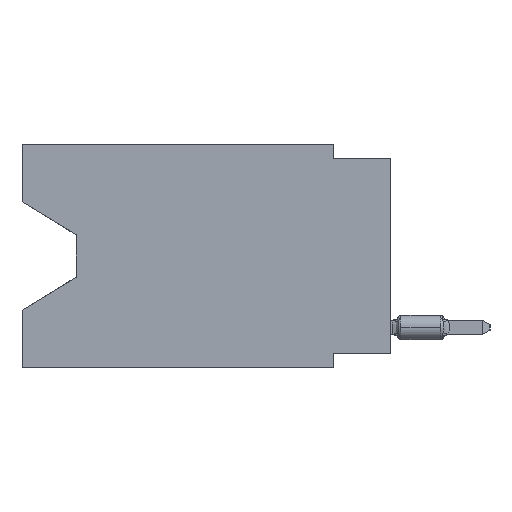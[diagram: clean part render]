
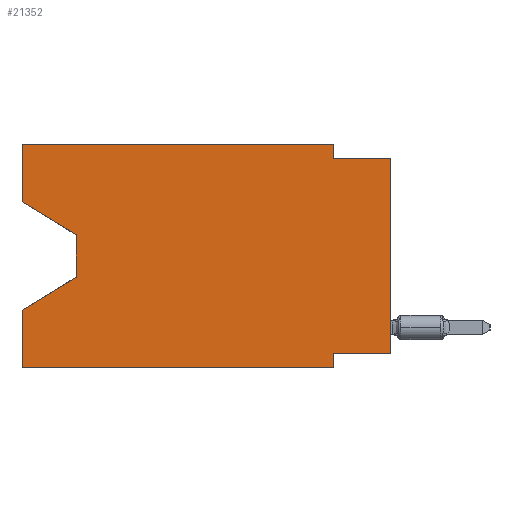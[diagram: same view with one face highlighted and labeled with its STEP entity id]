
A CAD part, left-side view. The second image highlights one B-rep face of the part: STEP entity #21352.
In plain terms, the highlighted planar face has unit normal (-1, 0, 0).
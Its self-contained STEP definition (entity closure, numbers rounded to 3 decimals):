
#1010 = VECTOR ( 'NONE', #30172, 1000. ) ;
#1150 = ORIENTED_EDGE ( 'NONE', *, *, #23051, .T. ) ;
#1176 = DIRECTION ( 'NONE',  ( 0., 0., 1. ) ) ;
#1302 = DIRECTION ( 'NONE',  ( 0., 0., 1. ) ) ;
#1735 = CARTESIAN_POINT ( 'NONE',  ( 0., 0., 0. ) ) ;
#2329 = EDGE_CURVE ( 'NONE', #19913, #29093, #39961, .T. ) ;
#2460 = CARTESIAN_POINT ( 'NONE',  ( 0., 16.383, -2.546 ) ) ;
#2605 = VERTEX_POINT ( 'NONE', #6800 ) ;
#3284 = VECTOR ( 'NONE', #35981, 1000. ) ;
#3631 = LINE ( 'NONE', #40760, #1010 ) ;
#3651 = CARTESIAN_POINT ( 'NONE',  ( 0., 2.54, 0. ) ) ;
#4094 = DIRECTION ( 'NONE',  ( 0., 1., 0. ) ) ;
#4139 = CARTESIAN_POINT ( 'NONE',  ( 0., 2.54, -9.906 ) ) ;
#4316 = VERTEX_POINT ( 'NONE', #26031 ) ;
#4637 = ORIENTED_EDGE ( 'NONE', *, *, #6625, .T. ) ;
#5094 = VECTOR ( 'NONE', #1302, 1000. ) ;
#5247 = EDGE_CURVE ( 'NONE', #20500, #32121, #35694, .T. ) ;
#6625 = EDGE_CURVE ( 'NONE', #19913, #32121, #41486, .T. ) ;
#6800 = CARTESIAN_POINT ( 'NONE',  ( 0., 16.383, -9.906 ) ) ;
#7264 = DIRECTION ( 'NONE',  ( 0., 0., -1. ) ) ;
#7619 = ORIENTED_EDGE ( 'NONE', *, *, #9772, .F. ) ;
#7693 = DIRECTION ( 'NONE',  ( 1., 0., 0. ) ) ;
#7771 = CARTESIAN_POINT ( 'NONE',  ( 0., 16.383, 0. ) ) ;
#7811 = LINE ( 'NONE', #4139, #41850 ) ;
#8236 = DIRECTION ( 'NONE',  ( 0., 0., 1. ) ) ;
#8363 = CARTESIAN_POINT ( 'NONE',  ( 0., 13.97, -5.893 ) ) ;
#8484 = EDGE_CURVE ( 'NONE', #26844, #34857, #31747, .T. ) ;
#8653 = CARTESIAN_POINT ( 'NONE',  ( 0., 16.383, 0. ) ) ;
#8928 = DIRECTION ( 'NONE',  ( 0., -1., 0. ) ) ;
#9772 = EDGE_CURVE ( 'NONE', #34857, #26220, #42355, .T. ) ;
#10543 = CARTESIAN_POINT ( 'NONE',  ( 0., 0., -0.635 ) ) ;
#11163 = LINE ( 'NONE', #14217, #24694 ) ;
#11628 = DIRECTION ( 'NONE',  ( 0., -0.855, -0.519 ) ) ;
#12392 = EDGE_CURVE ( 'NONE', #29044, #34066, #26334, .T. ) ;
#13186 = ORIENTED_EDGE ( 'NONE', *, *, #23347, .F. ) ;
#14217 = CARTESIAN_POINT ( 'NONE',  ( 0., 16.383, 0. ) ) ;
#14349 = EDGE_CURVE ( 'NONE', #2605, #34066, #11163, .T. ) ;
#15320 = CARTESIAN_POINT ( 'NONE',  ( 0., 2.54, -9.271 ) ) ;
#15843 = ORIENTED_EDGE ( 'NONE', *, *, #8484, .F. ) ;
#16494 = CARTESIAN_POINT ( 'NONE',  ( 0., 0., -9.271 ) ) ;
#17186 = ORIENTED_EDGE ( 'NONE', *, *, #35524, .T. ) ;
#17229 = ORIENTED_EDGE ( 'NONE', *, *, #12392, .T. ) ;
#17276 = FACE_OUTER_BOUND ( 'NONE', #36781, .T. ) ;
#17323 = VERTEX_POINT ( 'NONE', #34441 ) ;
#17388 = DIRECTION ( 'NONE',  ( 0., 0., -1. ) ) ;
#18300 = LINE ( 'NONE', #21785, #27297 ) ;
#18641 = EDGE_CURVE ( 'NONE', #26220, #20500, #3631, .T. ) ;
#19153 = ORIENTED_EDGE ( 'NONE', *, *, #14349, .F. ) ;
#19913 = VERTEX_POINT ( 'NONE', #31413 ) ;
#20136 = VECTOR ( 'NONE', #4094, 1000. ) ;
#20457 = ORIENTED_EDGE ( 'NONE', *, *, #18641, .F. ) ;
#20500 = VERTEX_POINT ( 'NONE', #32221 ) ;
#20895 = AXIS2_PLACEMENT_3D ( 'NONE', #30787, #7693, #7264 ) ;
#21352 = ADVANCED_FACE ( 'NONE', ( #17276 ), #37702, .F. ) ;
#21785 = CARTESIAN_POINT ( 'NONE',  ( 0., 16.383, -9.906 ) ) ;
#22021 = VECTOR ( 'NONE', #11628, 1000. ) ;
#22200 = CARTESIAN_POINT ( 'NONE',  ( 0., 16.383, 0. ) ) ;
#22385 = VECTOR ( 'NONE', #29401, 1000. ) ;
#22642 = DIRECTION ( 'NONE',  ( 0., 0.855, -0.519 ) ) ;
#22731 = LINE ( 'NONE', #36618, #3284 ) ;
#22875 = CARTESIAN_POINT ( 'NONE',  ( 0., 0., -0.635 ) ) ;
#23051 = EDGE_CURVE ( 'NONE', #2605, #17323, #18300, .T. ) ;
#23347 = EDGE_CURVE ( 'NONE', #29093, #17323, #7811, .T. ) ;
#24694 = VECTOR ( 'NONE', #1176, 1000. ) ;
#26031 = CARTESIAN_POINT ( 'NONE',  ( 0., 13.97, -4.013 ) ) ;
#26220 = VERTEX_POINT ( 'NONE', #3651 ) ;
#26334 = LINE ( 'NONE', #29168, #30709 ) ;
#26844 = VERTEX_POINT ( 'NONE', #2460 ) ;
#27297 = VECTOR ( 'NONE', #8928, 1000. ) ;
#29037 = LINE ( 'NONE', #34909, #22021 ) ;
#29044 = VERTEX_POINT ( 'NONE', #8363 ) ;
#29093 = VERTEX_POINT ( 'NONE', #15320 ) ;
#29168 = CARTESIAN_POINT ( 'NONE',  ( 0., 13.97, -5.893 ) ) ;
#29401 = DIRECTION ( 'NONE',  ( 0., -1., 0. ) ) ;
#29607 = VECTOR ( 'NONE', #35458, 1000. ) ;
#30172 = DIRECTION ( 'NONE',  ( 0., 0., -1. ) ) ;
#30709 = VECTOR ( 'NONE', #22642, 1000. ) ;
#30787 = CARTESIAN_POINT ( 'NONE',  ( 0., 16.383, 0. ) ) ;
#31413 = CARTESIAN_POINT ( 'NONE',  ( 0., 0., -9.271 ) ) ;
#31689 = ORIENTED_EDGE ( 'NONE', *, *, #5247, .F. ) ;
#31747 = LINE ( 'NONE', #8653, #5094 ) ;
#32121 = VERTEX_POINT ( 'NONE', #10543 ) ;
#32215 = VECTOR ( 'NONE', #8236, 1000. ) ;
#32221 = CARTESIAN_POINT ( 'NONE',  ( 0., 2.54, -0.635 ) ) ;
#33491 = ORIENTED_EDGE ( 'NONE', *, *, #35740, .T. ) ;
#33594 = ORIENTED_EDGE ( 'NONE', *, *, #2329, .F. ) ;
#34066 = VERTEX_POINT ( 'NONE', #34274 ) ;
#34274 = CARTESIAN_POINT ( 'NONE',  ( 0., 16.383, -7.36 ) ) ;
#34441 = CARTESIAN_POINT ( 'NONE',  ( 0., 2.54, -9.906 ) ) ;
#34857 = VERTEX_POINT ( 'NONE', #7771 ) ;
#34909 = CARTESIAN_POINT ( 'NONE',  ( 0., 16.383, -2.546 ) ) ;
#35458 = DIRECTION ( 'NONE',  ( 0., -1., 0. ) ) ;
#35524 = EDGE_CURVE ( 'NONE', #26844, #4316, #29037, .T. ) ;
#35694 = LINE ( 'NONE', #22875, #22385 ) ;
#35740 = EDGE_CURVE ( 'NONE', #4316, #29044, #22731, .T. ) ;
#35981 = DIRECTION ( 'NONE',  ( 0., 0., -1. ) ) ;
#36618 = CARTESIAN_POINT ( 'NONE',  ( 0., 13.97, -4.013 ) ) ;
#36781 = EDGE_LOOP ( 'NONE', ( #17186, #33491, #17229, #19153, #1150, #13186, #33594, #4637, #31689, #20457, #7619, #15843 ) ) ;
#37702 = PLANE ( 'NONE',  #20895 ) ;
#39961 = LINE ( 'NONE', #16494, #20136 ) ;
#40760 = CARTESIAN_POINT ( 'NONE',  ( 0., 2.54, 0. ) ) ;
#41486 = LINE ( 'NONE', #1735, #32215 ) ;
#41850 = VECTOR ( 'NONE', #17388, 1000. ) ;
#42355 = LINE ( 'NONE', #22200, #29607 ) ;
